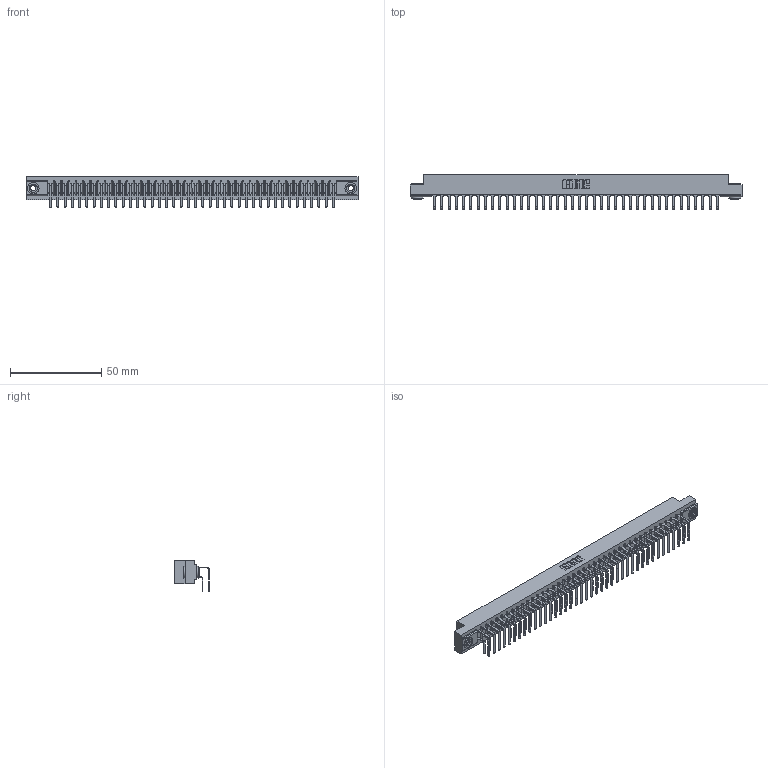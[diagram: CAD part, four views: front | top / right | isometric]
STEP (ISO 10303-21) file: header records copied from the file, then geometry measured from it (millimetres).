
FILE_DESCRIPTION (( 'STEP AP203' ), '1' );
FILE_NAME ('307-040-458-103.STEP', '2020-09-29T09:58:20', ( '' ), ( '' ), 'SwSTEP 2.0', 'SolidWorks 2020', '' );
FILE_SCHEMA (( 'CONFIG_CONTROL_DESIGN' ));
Length unit declared in the file: inch
Products named in the file (5): 307-040-458-103; 307-290-001_558 559 - 1 (Single); 307 Part_.156 Dia Mounting Holes; 345-250-002_345-250-002-102; 307-290-001_558 - 2 (Single)
Assembly tree (83 placements, depth 2):
  307-040-458-103
    307 Part_.156 Dia Mounting Holes
    307-290-001_558 559 - 1 (Single)  x40
    307-290-001_558 - 2 (Single)  x40
    345-250-002_345-250-002-102  x2
Bounding box: 181.51 x 18.96 x 16.8 mm (x, y, z)
Volume: 19643.1 mm3; surface area: 26310.6 mm2
Topology: 83 solids, 83 shells, 4211 faces, 11795 edges, 7642 vertices
Faces by surface type: plane 2734, cylinder 1387, sphere 82, cone 8
Entity records: 38330 total; most frequent: CARTESIAN_POINT 6255, ORIENTED_EDGE 6190, DIRECTION 6141, EDGE_CURVE 3095, LINE 2365, VECTOR 2365, VERTEX_POINT 2002, AXIS2_PLACEMENT_3D 1888
